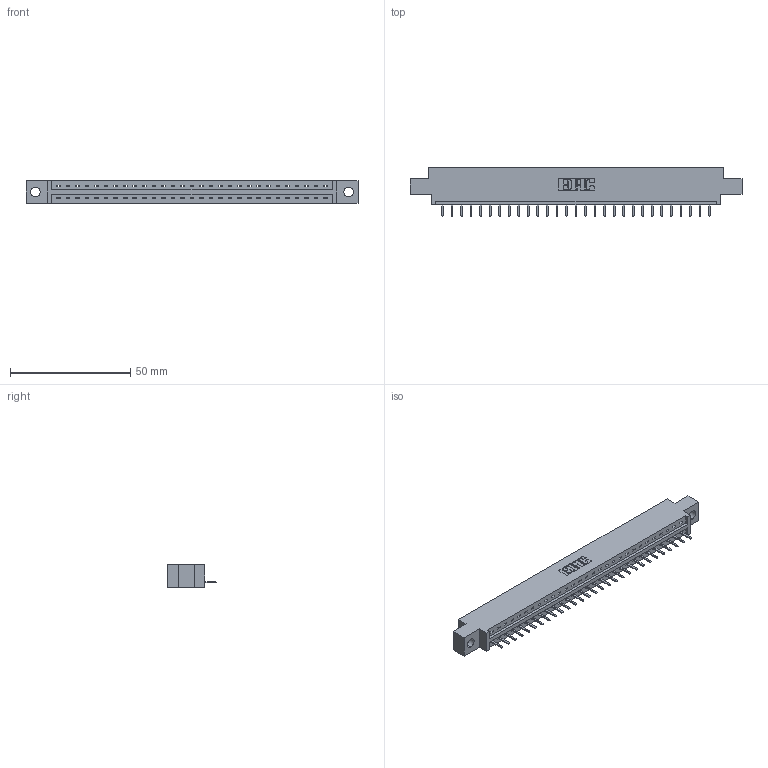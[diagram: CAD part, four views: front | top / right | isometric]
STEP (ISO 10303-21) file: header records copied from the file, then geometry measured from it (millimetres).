
FILE_DESCRIPTION (( 'STEP AP203' ), '1' );
FILE_NAME ('387-029-520-604.STEP', '2018-09-17T00:54:15', ( '' ), ( '' ), 'SwSTEP 2.0', 'SolidWorks 2016', '' );
FILE_SCHEMA (( 'CONFIG_CONTROL_DESIGN' ));
Length unit declared in the file: inch
Products named in the file (3): 345-292-001_345-293-120; 387-029-520-604; 337 Part_0.170 Offset - 0.156 Dia-TH
Assembly tree (30 placements, depth 2):
  387-029-520-604
    337 Part_0.170 Offset - 0.156 Dia-TH
    345-292-001_345-293-120  x29
Bounding box: 137.92 x 20.02 x 9.4 mm (x, y, z)
Volume: 13883.2 mm3; surface area: 13865.5 mm2
Topology: 30 solids, 30 shells, 2032 faces, 6007 edges, 3926 vertices
Faces by surface type: plane 1466, cylinder 566
Entity records: 23487 total; most frequent: CARTESIAN_POINT 4109, ORIENTED_EDGE 4062, DIRECTION 3473, EDGE_CURVE 2031, VECTOR 1899, LINE 1899, VERTEX_POINT 1350, AXIS2_PLACEMENT_3D 787
